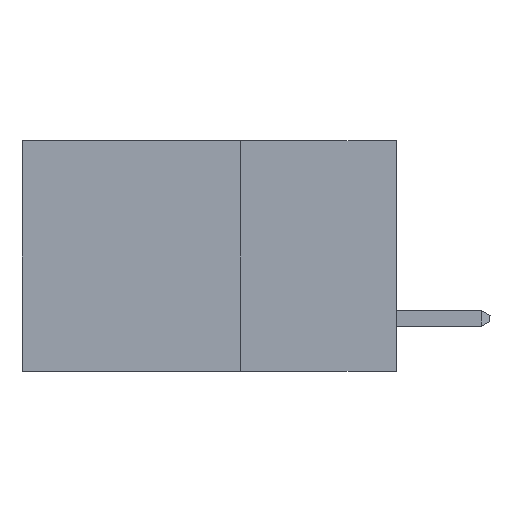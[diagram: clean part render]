
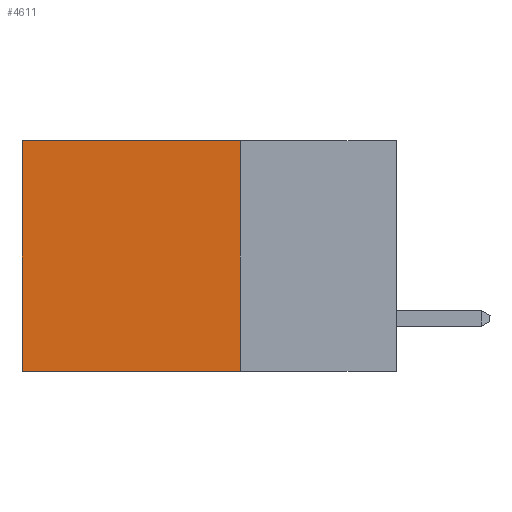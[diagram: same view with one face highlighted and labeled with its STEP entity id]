
A CAD part, left-side view. The second image highlights one B-rep face of the part: STEP entity #4611.
In plain terms, the highlighted planar face has unit normal (-1, 0, 0).
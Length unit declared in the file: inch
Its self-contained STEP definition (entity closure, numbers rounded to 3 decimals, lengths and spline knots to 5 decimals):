
#336 = DIRECTION ( 'NONE',  ( 1., 0., 0. ) ) ;
#1193 = VERTEX_POINT ( 'NONE', #3471 ) ;
#1553 = EDGE_CURVE ( 'NONE', #16366, #7573, #3093, .T. ) ;
#2268 = CARTESIAN_POINT ( 'NONE',  ( 0.2615, 0.25, -0.37 ) ) ;
#2380 = VECTOR ( 'NONE', #15549, 39.37008 ) ;
#2509 = DIRECTION ( 'NONE',  ( 0., 1., 0. ) ) ;
#3093 = LINE ( 'NONE', #4980, #2380 ) ;
#3471 = CARTESIAN_POINT ( 'NONE',  ( 0.2615, 0.25, 0. ) ) ;
#4611 = ADVANCED_FACE ( 'NONE', ( #9449 ), #20252, .F. ) ;
#4910 = VECTOR ( 'NONE', #18157, 39.37008 ) ;
#4980 = CARTESIAN_POINT ( 'NONE',  ( 0.2615, 0.6, -0.37 ) ) ;
#5444 = ORIENTED_EDGE ( 'NONE', *, *, #15359, .T. ) ;
#6163 = CARTESIAN_POINT ( 'NONE',  ( 0.2615, 0.25, 0. ) ) ;
#6471 = AXIS2_PLACEMENT_3D ( 'NONE', #11412, #336, #7471 ) ;
#7005 = DIRECTION ( 'NONE',  ( 0., 0., -1. ) ) ;
#7056 = EDGE_CURVE ( 'NONE', #1193, #17690, #19106, .T. ) ;
#7471 = DIRECTION ( 'NONE',  ( 0., 0., -1. ) ) ;
#7573 = VERTEX_POINT ( 'NONE', #14732 ) ;
#8522 = ORIENTED_EDGE ( 'NONE', *, *, #7056, .F. ) ;
#9449 = FACE_OUTER_BOUND ( 'NONE', #19907, .T. ) ;
#10488 = CARTESIAN_POINT ( 'NONE',  ( 0.2615, 0.6, 0. ) ) ;
#11412 = CARTESIAN_POINT ( 'NONE',  ( 0.2615, 0.25, -0.37 ) ) ;
#11977 = VECTOR ( 'NONE', #7005, 39.37008 ) ;
#13246 = LINE ( 'NONE', #6163, #4910 ) ;
#14273 = EDGE_CURVE ( 'NONE', #17690, #7573, #18580, .T. ) ;
#14732 = CARTESIAN_POINT ( 'NONE',  ( 0.2615, 0.6, -0.37 ) ) ;
#15287 = CARTESIAN_POINT ( 'NONE',  ( 0.2615, 0.25, -0.37 ) ) ;
#15359 = EDGE_CURVE ( 'NONE', #1193, #16366, #13246, .T. ) ;
#15549 = DIRECTION ( 'NONE',  ( 0., 0., -1. ) ) ;
#15644 = VECTOR ( 'NONE', #2509, 39.37008 ) ;
#15738 = CARTESIAN_POINT ( 'NONE',  ( 0.2615, 0.25, -0.37 ) ) ;
#16366 = VERTEX_POINT ( 'NONE', #10488 ) ;
#17587 = ORIENTED_EDGE ( 'NONE', *, *, #1553, .T. ) ;
#17690 = VERTEX_POINT ( 'NONE', #15287 ) ;
#18157 = DIRECTION ( 'NONE',  ( 0., 1., 0. ) ) ;
#18580 = LINE ( 'NONE', #2268, #15644 ) ;
#19106 = LINE ( 'NONE', #15738, #11977 ) ;
#19312 = ORIENTED_EDGE ( 'NONE', *, *, #14273, .F. ) ;
#19907 = EDGE_LOOP ( 'NONE', ( #17587, #19312, #8522, #5444 ) ) ;
#20252 = PLANE ( 'NONE',  #6471 ) ;
